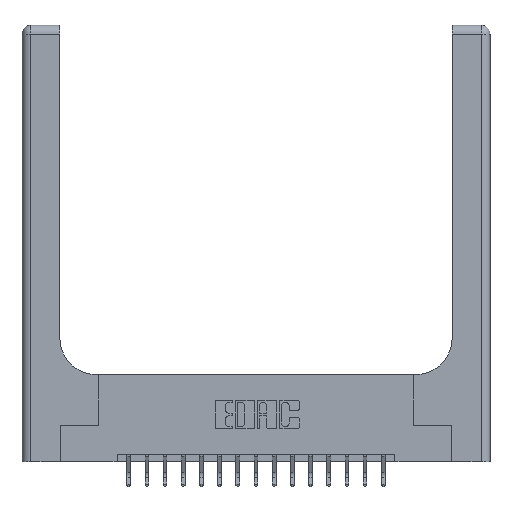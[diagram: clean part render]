
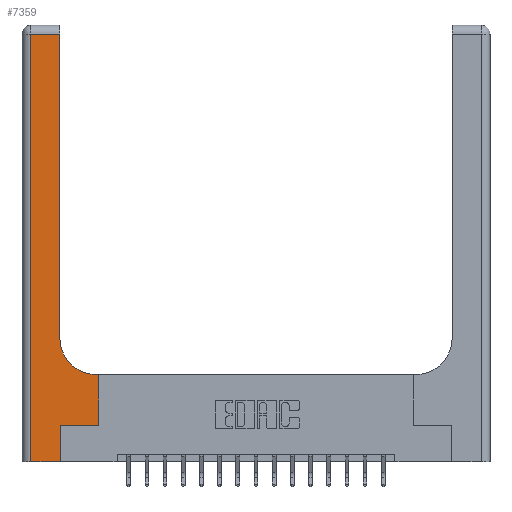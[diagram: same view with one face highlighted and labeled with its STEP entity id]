
A CAD part, top view. The second image highlights one B-rep face of the part: STEP entity #7359.
In plain terms, the highlighted planar face has unit normal (0, 0, 1).
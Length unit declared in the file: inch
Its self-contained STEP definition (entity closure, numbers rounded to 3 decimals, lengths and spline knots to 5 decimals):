
#111 = FACE_OUTER_BOUND ( 'NONE', #12950, .T. ) ;
#134 = DIRECTION ( 'NONE',  ( 1., 0., 0. ) ) ;
#296 = CARTESIAN_POINT ( 'NONE',  ( 0.528, 0.25, 0.37 ) ) ;
#522 = CARTESIAN_POINT ( 'NONE',  ( 0.265, 0., 0.37 ) ) ;
#562 = VERTEX_POINT ( 'NONE', #1706 ) ;
#1427 = LINE ( 'NONE', #296, #17598 ) ;
#1706 = CARTESIAN_POINT ( 'NONE',  ( 0.265, 0.25, 0.37 ) ) ;
#2032 = DIRECTION ( 'NONE',  ( 0., 1., 0. ) ) ;
#2221 = CARTESIAN_POINT ( 'NONE',  ( 0.26, 0.6, 0.37 ) ) ;
#2739 = VERTEX_POINT ( 'NONE', #15850 ) ;
#2901 = VECTOR ( 'NONE', #11956, 39.37008 ) ;
#4185 = EDGE_CURVE ( 'NONE', #5968, #562, #5866, .T. ) ;
#4626 = LINE ( 'NONE', #5640, #7135 ) ;
#5027 = DIRECTION ( 'NONE',  ( 0., 0., -1. ) ) ;
#5344 = VERTEX_POINT ( 'NONE', #17780 ) ;
#5488 = VERTEX_POINT ( 'NONE', #7619 ) ;
#5555 = VERTEX_POINT ( 'NONE', #14652 ) ;
#5640 = CARTESIAN_POINT ( 'NONE',  ( 0.06, 3., 0.37 ) ) ;
#5866 = LINE ( 'NONE', #522, #2901 ) ;
#5968 = VERTEX_POINT ( 'NONE', #8827 ) ;
#6468 = LINE ( 'NONE', #10086, #14667 ) ;
#6611 = CARTESIAN_POINT ( 'NONE',  ( 0., 2.94, 0.37 ) ) ;
#6613 = CARTESIAN_POINT ( 'NONE',  ( 0.51, 0.85, 0.37 ) ) ;
#6656 = DIRECTION ( 'NONE',  ( 1., 0., 0. ) ) ;
#6696 = EDGE_CURVE ( 'NONE', #5555, #16466, #10333, .T. ) ;
#6711 = LINE ( 'NONE', #2221, #13567 ) ;
#6789 = VECTOR ( 'NONE', #6656, 39.37008 ) ;
#6863 = EDGE_CURVE ( 'NONE', #5344, #2739, #6711, .T. ) ;
#7135 = VECTOR ( 'NONE', #11175, 39.37008 ) ;
#7159 = CARTESIAN_POINT ( 'NONE',  ( 0.26, 2.94, 0.37 ) ) ;
#7359 = ADVANCED_FACE ( 'NONE', ( #111 ), #13789, .F. ) ;
#7619 = CARTESIAN_POINT ( 'NONE',  ( 0.06, 0., 0.37 ) ) ;
#7662 = EDGE_CURVE ( 'NONE', #5488, #5968, #6468, .T. ) ;
#8503 = ORIENTED_EDGE ( 'NONE', *, *, #7662, .T. ) ;
#8827 = CARTESIAN_POINT ( 'NONE',  ( 0.265, 0., 0.37 ) ) ;
#9098 = CARTESIAN_POINT ( 'NONE',  ( 0.06, 2.94, 0.37 ) ) ;
#9459 = AXIS2_PLACEMENT_3D ( 'NONE', #11065, #5027, #11002 ) ;
#9725 = ORIENTED_EDGE ( 'NONE', *, *, #15833, .T. ) ;
#10086 = CARTESIAN_POINT ( 'NONE',  ( 0., 0., 0.37 ) ) ;
#10333 = LINE ( 'NONE', #11506, #17665 ) ;
#10367 = VERTEX_POINT ( 'NONE', #12368 ) ;
#10804 = AXIS2_PLACEMENT_3D ( 'NONE', #6613, #14074, #15475 ) ;
#11002 = DIRECTION ( 'NONE',  ( -1., 0., 0. ) ) ;
#11065 = CARTESIAN_POINT ( 'NONE',  ( 0., 3., 0.37 ) ) ;
#11114 = LINE ( 'NONE', #18195, #6789 ) ;
#11175 = DIRECTION ( 'NONE',  ( 0., -1., 0. ) ) ;
#11506 = CARTESIAN_POINT ( 'NONE',  ( 0.26, 3., 0.37 ) ) ;
#11745 = ORIENTED_EDGE ( 'NONE', *, *, #14510, .T. ) ;
#11882 = EDGE_CURVE ( 'NONE', #16466, #16520, #14506, .T. ) ;
#11956 = DIRECTION ( 'NONE',  ( 0., 1., 0. ) ) ;
#11985 = DIRECTION ( 'NONE',  ( 0., 1., 0. ) ) ;
#12368 = CARTESIAN_POINT ( 'NONE',  ( 0.528, 0.25, 0.37 ) ) ;
#12405 = DIRECTION ( 'NONE',  ( -1., 0., 0. ) ) ;
#12950 = EDGE_LOOP ( 'NONE', ( #14881, #17765, #16204, #8503, #15418, #9725, #11745, #18494, #17131 ) ) ;
#13567 = VECTOR ( 'NONE', #12405, 39.37008 ) ;
#13630 = EDGE_CURVE ( 'NONE', #16520, #5488, #4626, .T. ) ;
#13789 = PLANE ( 'NONE',  #9459 ) ;
#14074 = DIRECTION ( 'NONE',  ( 0., 0., -1. ) ) ;
#14506 = LINE ( 'NONE', #6611, #15877 ) ;
#14510 = EDGE_CURVE ( 'NONE', #10367, #5344, #1427, .T. ) ;
#14652 = CARTESIAN_POINT ( 'NONE',  ( 0.26, 0.85, 0.37 ) ) ;
#14667 = VECTOR ( 'NONE', #134, 39.37008 ) ;
#14881 = ORIENTED_EDGE ( 'NONE', *, *, #6696, .T. ) ;
#15418 = ORIENTED_EDGE ( 'NONE', *, *, #4185, .T. ) ;
#15475 = DIRECTION ( 'NONE',  ( 1., 0., 0. ) ) ;
#15833 = EDGE_CURVE ( 'NONE', #562, #10367, #11114, .T. ) ;
#15850 = CARTESIAN_POINT ( 'NONE',  ( 0.51, 0.6, 0.37 ) ) ;
#15877 = VECTOR ( 'NONE', #16808, 39.37008 ) ;
#16204 = ORIENTED_EDGE ( 'NONE', *, *, #13630, .T. ) ;
#16466 = VERTEX_POINT ( 'NONE', #7159 ) ;
#16519 = CIRCLE ( 'NONE', #10804, 0.25 ) ;
#16520 = VERTEX_POINT ( 'NONE', #9098 ) ;
#16808 = DIRECTION ( 'NONE',  ( -1., 0., 0. ) ) ;
#17131 = ORIENTED_EDGE ( 'NONE', *, *, #18041, .T. ) ;
#17598 = VECTOR ( 'NONE', #11985, 39.37008 ) ;
#17665 = VECTOR ( 'NONE', #2032, 39.37008 ) ;
#17765 = ORIENTED_EDGE ( 'NONE', *, *, #11882, .T. ) ;
#17780 = CARTESIAN_POINT ( 'NONE',  ( 0.528, 0.6, 0.37 ) ) ;
#18041 = EDGE_CURVE ( 'NONE', #2739, #5555, #16519, .T. ) ;
#18195 = CARTESIAN_POINT ( 'NONE',  ( 0.265, 0.25, 0.37 ) ) ;
#18494 = ORIENTED_EDGE ( 'NONE', *, *, #6863, .T. ) ;
